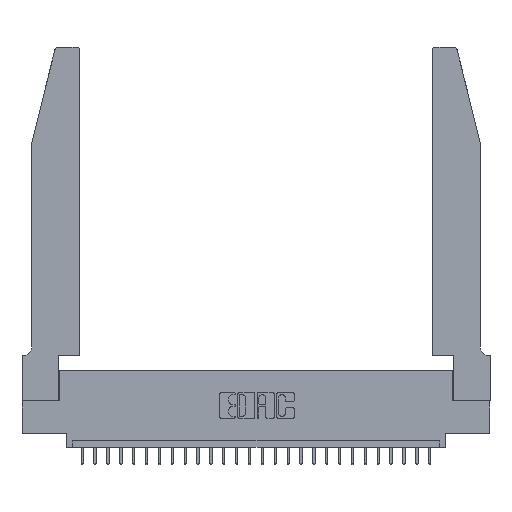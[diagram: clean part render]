
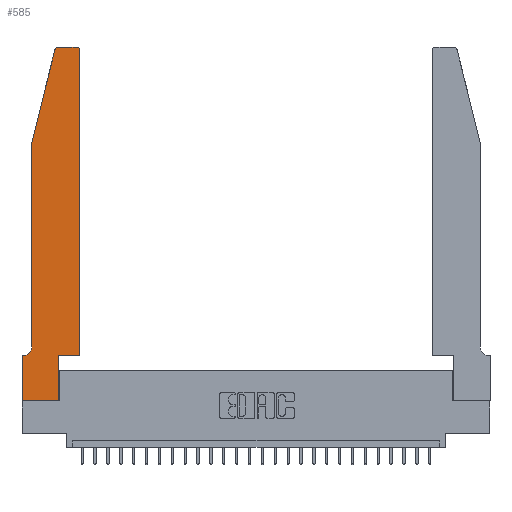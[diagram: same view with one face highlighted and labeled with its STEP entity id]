
A CAD part, top view. The second image highlights one B-rep face of the part: STEP entity #585.
In plain terms, the highlighted planar face has unit normal (0, 0, 1).
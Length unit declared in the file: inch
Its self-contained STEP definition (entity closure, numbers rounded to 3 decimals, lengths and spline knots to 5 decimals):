
#376 = VERTEX_POINT ( 'NONE', #10370 ) ;
#460 = DIRECTION ( 'NONE',  ( 1., 0., 0. ) ) ;
#585 = ADVANCED_FACE ( 'NONE', ( #13453 ), #17960, .T. ) ;
#1265 = LINE ( 'NONE', #9855, #19390 ) ;
#1305 = VECTOR ( 'NONE', #23330, 39.37008 ) ;
#1460 = DIRECTION ( 'NONE',  ( 0., 0., 1. ) ) ;
#1595 = DIRECTION ( 'NONE',  ( 1., 0., 0. ) ) ;
#1762 = EDGE_LOOP ( 'NONE', ( #15397, #23786, #19812, #8639, #26643, #26912, #17904, #5616, #27469, #20389, #2151, #27838 ) ) ;
#2151 = ORIENTED_EDGE ( 'NONE', *, *, #26345, .T. ) ;
#2376 = CARTESIAN_POINT ( 'NONE',  ( 0.0755, 0.35, 0.37 ) ) ;
#3217 = EDGE_CURVE ( 'NONE', #23253, #16080, #3466, .T. ) ;
#3466 = LINE ( 'NONE', #16443, #19590 ) ;
#3677 = CARTESIAN_POINT ( 'NONE',  ( 0.0755, 2., 0.37 ) ) ;
#3684 = CARTESIAN_POINT ( 'NONE',  ( 0., 0., 0.37 ) ) ;
#3964 = VERTEX_POINT ( 'NONE', #15504 ) ;
#4156 = VERTEX_POINT ( 'NONE', #16340 ) ;
#4568 = VERTEX_POINT ( 'NONE', #5158 ) ;
#4931 = CARTESIAN_POINT ( 'NONE',  ( 0.0055, 0.35, 0.37 ) ) ;
#5158 = CARTESIAN_POINT ( 'NONE',  ( 0.284, 2.75, 0.37 ) ) ;
#5388 = LINE ( 'NONE', #9893, #5837 ) ;
#5612 = VERTEX_POINT ( 'NONE', #10874 ) ;
#5616 = ORIENTED_EDGE ( 'NONE', *, *, #11230, .T. ) ;
#5650 = CARTESIAN_POINT ( 'NONE',  ( 0.4505, 0.35, 0.37 ) ) ;
#5837 = VECTOR ( 'NONE', #18513, 39.37008 ) ;
#6452 = VECTOR ( 'NONE', #20002, 39.37008 ) ;
#6949 = DIRECTION ( 'NONE',  ( 0., 0., 1. ) ) ;
#7022 = VERTEX_POINT ( 'NONE', #15253 ) ;
#7108 = CARTESIAN_POINT ( 'NONE',  ( 0.4205, 2.72, 0.37 ) ) ;
#7570 = CIRCLE ( 'NONE', #9847, 0.03 ) ;
#8384 = AXIS2_PLACEMENT_3D ( 'NONE', #7108, #9364, #18265 ) ;
#8464 = LINE ( 'NONE', #10472, #26688 ) ;
#8639 = ORIENTED_EDGE ( 'NONE', *, *, #3217, .T. ) ;
#9364 = DIRECTION ( 'NONE',  ( 0., 0., 1. ) ) ;
#9827 = CARTESIAN_POINT ( 'NONE',  ( 0., 0.35, 0.37 ) ) ;
#9847 = AXIS2_PLACEMENT_3D ( 'NONE', #16688, #1460, #1595 ) ;
#9855 = CARTESIAN_POINT ( 'NONE',  ( 0.2865, 0.35, 0.37 ) ) ;
#9893 = CARTESIAN_POINT ( 'NONE',  ( 0., 0., 0.37 ) ) ;
#10370 = CARTESIAN_POINT ( 'NONE',  ( 0.4505, 0.35, 0.37 ) ) ;
#10472 = CARTESIAN_POINT ( 'NONE',  ( 0.0755, 2., 0.37 ) ) ;
#10874 = CARTESIAN_POINT ( 'NONE',  ( 0., 0., 0.37 ) ) ;
#11056 = DIRECTION ( 'NONE',  ( -1., 0., 0. ) ) ;
#11230 = EDGE_CURVE ( 'NONE', #5612, #17908, #5388, .T. ) ;
#11622 = DIRECTION ( 'NONE',  ( 1., 0., 0. ) ) ;
#12090 = EDGE_CURVE ( 'NONE', #17908, #27603, #1265, .T. ) ;
#12274 = CARTESIAN_POINT ( 'NONE',  ( 0.2865, 0.35, 0.37 ) ) ;
#13058 = VERTEX_POINT ( 'NONE', #4931 ) ;
#13095 = LINE ( 'NONE', #2376, #6452 ) ;
#13212 = LINE ( 'NONE', #24115, #19446 ) ;
#13308 = LINE ( 'NONE', #23664, #18298 ) ;
#13453 = FACE_OUTER_BOUND ( 'NONE', #1762, .T. ) ;
#13702 = VERTEX_POINT ( 'NONE', #9827 ) ;
#14263 = DIRECTION ( 'NONE',  ( 0., 1., 0. ) ) ;
#14330 = DIRECTION ( 'NONE',  ( 0., -1., 0. ) ) ;
#15090 = EDGE_CURVE ( 'NONE', #4156, #4568, #13212, .T. ) ;
#15253 = CARTESIAN_POINT ( 'NONE',  ( 0.25487, 2.72718, 0.37 ) ) ;
#15397 = ORIENTED_EDGE ( 'NONE', *, *, #15090, .T. ) ;
#15504 = CARTESIAN_POINT ( 'NONE',  ( 0.4505, 2.72, 0.37 ) ) ;
#15882 = AXIS2_PLACEMENT_3D ( 'NONE', #19656, #19380, #11056 ) ;
#16080 = VERTEX_POINT ( 'NONE', #26016 ) ;
#16340 = CARTESIAN_POINT ( 'NONE',  ( 0.4205, 2.75, 0.37 ) ) ;
#16443 = CARTESIAN_POINT ( 'NONE',  ( 0.0755, 2., 0.37 ) ) ;
#16688 = CARTESIAN_POINT ( 'NONE',  ( 0.284, 2.72, 0.37 ) ) ;
#16928 = EDGE_CURVE ( 'NONE', #16080, #13058, #17705, .T. ) ;
#17126 = VECTOR ( 'NONE', #14263, 39.37008 ) ;
#17231 = DIRECTION ( 'NONE',  ( -0.239, -0.971, 0. ) ) ;
#17705 = CIRCLE ( 'NONE', #15882, 0.07 ) ;
#17722 = EDGE_CURVE ( 'NONE', #13058, #13702, #13095, .T. ) ;
#17904 = ORIENTED_EDGE ( 'NONE', *, *, #24939, .T. ) ;
#17908 = VERTEX_POINT ( 'NONE', #19386 ) ;
#17960 = PLANE ( 'NONE',  #26366 ) ;
#18265 = DIRECTION ( 'NONE',  ( 1., 0., 0. ) ) ;
#18298 = VECTOR ( 'NONE', #460, 39.37008 ) ;
#18513 = DIRECTION ( 'NONE',  ( 1., 0., 0. ) ) ;
#19220 = CIRCLE ( 'NONE', #8384, 0.03 ) ;
#19380 = DIRECTION ( 'NONE',  ( 0., 0., -1. ) ) ;
#19386 = CARTESIAN_POINT ( 'NONE',  ( 0.2865, 0., 0.37 ) ) ;
#19390 = VECTOR ( 'NONE', #22879, 39.37008 ) ;
#19446 = VECTOR ( 'NONE', #27938, 39.37008 ) ;
#19590 = VECTOR ( 'NONE', #14330, 39.37008 ) ;
#19656 = CARTESIAN_POINT ( 'NONE',  ( 0.0055, 0.42, 0.37 ) ) ;
#19812 = ORIENTED_EDGE ( 'NONE', *, *, #27302, .T. ) ;
#20002 = DIRECTION ( 'NONE',  ( -1., 0., 0. ) ) ;
#20389 = ORIENTED_EDGE ( 'NONE', *, *, #22102, .T. ) ;
#20609 = EDGE_CURVE ( 'NONE', #3964, #4156, #19220, .T. ) ;
#22102 = EDGE_CURVE ( 'NONE', #27603, #376, #13308, .T. ) ;
#22879 = DIRECTION ( 'NONE',  ( 0., 1., 0. ) ) ;
#23041 = LINE ( 'NONE', #3684, #1305 ) ;
#23253 = VERTEX_POINT ( 'NONE', #3677 ) ;
#23330 = DIRECTION ( 'NONE',  ( 0., -1., 0. ) ) ;
#23664 = CARTESIAN_POINT ( 'NONE',  ( 0.4505, 0.35, 0.37 ) ) ;
#23786 = ORIENTED_EDGE ( 'NONE', *, *, #24669, .T. ) ;
#24115 = CARTESIAN_POINT ( 'NONE',  ( 0.2605, 2.75, 0.37 ) ) ;
#24669 = EDGE_CURVE ( 'NONE', #4568, #7022, #7570, .T. ) ;
#24939 = EDGE_CURVE ( 'NONE', #13702, #5612, #23041, .T. ) ;
#25038 = LINE ( 'NONE', #5650, #17126 ) ;
#26016 = CARTESIAN_POINT ( 'NONE',  ( 0.0755, 0.42, 0.37 ) ) ;
#26345 = EDGE_CURVE ( 'NONE', #376, #3964, #25038, .T. ) ;
#26357 = CARTESIAN_POINT ( 'NONE',  ( 0., 0.35, 0.37 ) ) ;
#26366 = AXIS2_PLACEMENT_3D ( 'NONE', #26357, #6949, #11622 ) ;
#26643 = ORIENTED_EDGE ( 'NONE', *, *, #16928, .T. ) ;
#26688 = VECTOR ( 'NONE', #17231, 39.37008 ) ;
#26912 = ORIENTED_EDGE ( 'NONE', *, *, #17722, .T. ) ;
#27302 = EDGE_CURVE ( 'NONE', #7022, #23253, #8464, .T. ) ;
#27469 = ORIENTED_EDGE ( 'NONE', *, *, #12090, .T. ) ;
#27603 = VERTEX_POINT ( 'NONE', #12274 ) ;
#27838 = ORIENTED_EDGE ( 'NONE', *, *, #20609, .T. ) ;
#27938 = DIRECTION ( 'NONE',  ( -1., 0., 0. ) ) ;
